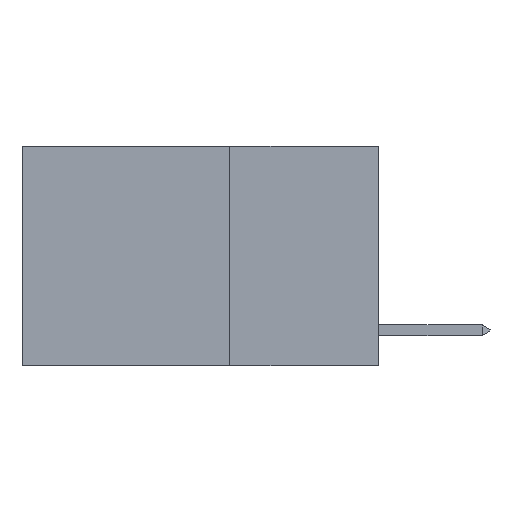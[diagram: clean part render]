
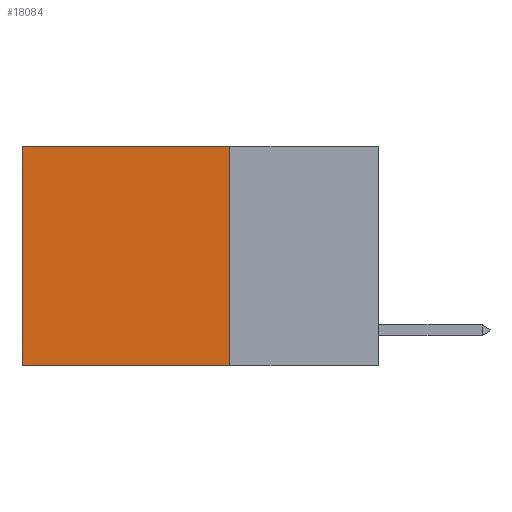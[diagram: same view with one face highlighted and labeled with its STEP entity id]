
A CAD part, left-side view. The second image highlights one B-rep face of the part: STEP entity #18084.
In plain terms, the highlighted planar face has unit normal (-1, 0, 0).
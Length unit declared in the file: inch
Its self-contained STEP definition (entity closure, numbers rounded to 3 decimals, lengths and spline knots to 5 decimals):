
#3939 = VERTEX_POINT ( 'NONE', #7313 ) ;
#4616 = VECTOR ( 'NONE', #22683, 39.37008 ) ;
#4948 = ORIENTED_EDGE ( 'NONE', *, *, #14464, .T. ) ;
#5092 = ORIENTED_EDGE ( 'NONE', *, *, #10770, .T. ) ;
#5152 = LINE ( 'NONE', #15752, #21621 ) ;
#5164 = VECTOR ( 'NONE', #8218, 39.37008 ) ;
#6180 = CARTESIAN_POINT ( 'NONE',  ( 0.2625, 0.6, 0. ) ) ;
#6299 = AXIS2_PLACEMENT_3D ( 'NONE', #23599, #11220, #25629 ) ;
#7108 = PLANE ( 'NONE',  #6299 ) ;
#7313 = CARTESIAN_POINT ( 'NONE',  ( 0.2625, 0.25, 0. ) ) ;
#7522 = VERTEX_POINT ( 'NONE', #14066 ) ;
#7604 = DIRECTION ( 'NONE',  ( 0., 0., -1. ) ) ;
#7735 = CARTESIAN_POINT ( 'NONE',  ( 0.2625, 0.6, 0. ) ) ;
#8218 = DIRECTION ( 'NONE',  ( 0., 1., 0. ) ) ;
#8665 = DIRECTION ( 'NONE',  ( 0., 1., 0. ) ) ;
#10661 = LINE ( 'NONE', #18525, #5164 ) ;
#10749 = LINE ( 'NONE', #6180, #4616 ) ;
#10770 = EDGE_CURVE ( 'NONE', #15637, #7522, #10749, .T. ) ;
#11220 = DIRECTION ( 'NONE',  ( 1., 0., 0. ) ) ;
#14066 = CARTESIAN_POINT ( 'NONE',  ( 0.2625, 0.6, -0.37 ) ) ;
#14335 = EDGE_CURVE ( 'NONE', #15145, #7522, #10661, .T. ) ;
#14464 = EDGE_CURVE ( 'NONE', #3939, #15637, #18144, .T. ) ;
#15145 = VERTEX_POINT ( 'NONE', #20479 ) ;
#15637 = VERTEX_POINT ( 'NONE', #7735 ) ;
#15752 = CARTESIAN_POINT ( 'NONE',  ( 0.2625, 0.25, 0. ) ) ;
#16515 = FACE_OUTER_BOUND ( 'NONE', #18710, .T. ) ;
#18084 = ADVANCED_FACE ( 'NONE', ( #16515 ), #7108, .F. ) ;
#18144 = LINE ( 'NONE', #21010, #23612 ) ;
#18525 = CARTESIAN_POINT ( 'NONE',  ( 0.2625, 0.25, -0.37 ) ) ;
#18680 = ORIENTED_EDGE ( 'NONE', *, *, #14335, .F. ) ;
#18710 = EDGE_LOOP ( 'NONE', ( #5092, #18680, #22527, #4948 ) ) ;
#20479 = CARTESIAN_POINT ( 'NONE',  ( 0.2625, 0.25, -0.37 ) ) ;
#21010 = CARTESIAN_POINT ( 'NONE',  ( 0.2625, 0.25, 0. ) ) ;
#21621 = VECTOR ( 'NONE', #7604, 39.37008 ) ;
#22527 = ORIENTED_EDGE ( 'NONE', *, *, #24356, .F. ) ;
#22683 = DIRECTION ( 'NONE',  ( 0., 0., -1. ) ) ;
#23599 = CARTESIAN_POINT ( 'NONE',  ( 0.2625, 0.25, 0. ) ) ;
#23612 = VECTOR ( 'NONE', #8665, 39.37008 ) ;
#24356 = EDGE_CURVE ( 'NONE', #3939, #15145, #5152, .T. ) ;
#25629 = DIRECTION ( 'NONE',  ( 0., 0., -1. ) ) ;
